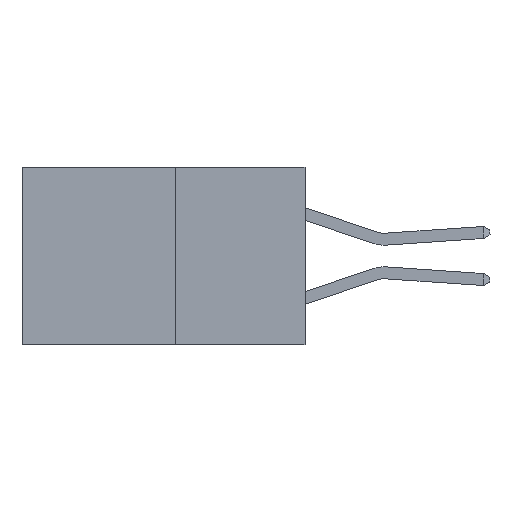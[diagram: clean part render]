
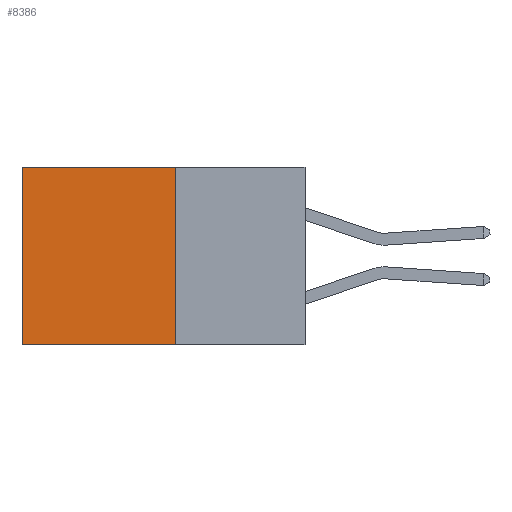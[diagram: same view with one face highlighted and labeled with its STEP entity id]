
A CAD part, left-side view. The second image highlights one B-rep face of the part: STEP entity #8386.
In plain terms, the highlighted planar face has unit normal (-1, 0, 0).
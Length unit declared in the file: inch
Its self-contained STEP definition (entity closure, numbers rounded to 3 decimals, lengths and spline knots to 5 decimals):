
#73 = CARTESIAN_POINT ( 'NONE',  ( 0.277, 0.27, -0.37 ) ) ;
#187 = DIRECTION ( 'NONE',  ( 0., 0., -1. ) ) ;
#1354 = EDGE_CURVE ( 'NONE', #4958, #6235, #5402, .T. ) ;
#1986 = EDGE_CURVE ( 'NONE', #6235, #6941, #6655, .T. ) ;
#2369 = CARTESIAN_POINT ( 'NONE',  ( 0.277, 0.27, -0.37 ) ) ;
#2407 = VECTOR ( 'NONE', #4688, 39.37008 ) ;
#2546 = EDGE_LOOP ( 'NONE', ( #6304, #5049, #4084, #9628 ) ) ;
#2967 = CARTESIAN_POINT ( 'NONE',  ( 0.277, 0.27, 0. ) ) ;
#3850 = CARTESIAN_POINT ( 'NONE',  ( 0.277, 0.27, -0.37 ) ) ;
#3928 = EDGE_CURVE ( 'NONE', #4958, #4453, #10139, .T. ) ;
#3940 = AXIS2_PLACEMENT_3D ( 'NONE', #2369, #4893, #10057 ) ;
#4017 = CARTESIAN_POINT ( 'NONE',  ( 0.277, 0.59, -0.37 ) ) ;
#4084 = ORIENTED_EDGE ( 'NONE', *, *, #1354, .F. ) ;
#4098 = DIRECTION ( 'NONE',  ( 0., 0., -1. ) ) ;
#4453 = VERTEX_POINT ( 'NONE', #5354 ) ;
#4454 = VECTOR ( 'NONE', #7795, 39.37008 ) ;
#4688 = DIRECTION ( 'NONE',  ( 0., 1., 0. ) ) ;
#4707 = EDGE_CURVE ( 'NONE', #4453, #6941, #5083, .T. ) ;
#4893 = DIRECTION ( 'NONE',  ( 1., 0., 0. ) ) ;
#4958 = VERTEX_POINT ( 'NONE', #2967 ) ;
#5049 = ORIENTED_EDGE ( 'NONE', *, *, #1986, .F. ) ;
#5083 = LINE ( 'NONE', #4017, #5330 ) ;
#5199 = CARTESIAN_POINT ( 'NONE',  ( 0.277, 0.27, -0.37 ) ) ;
#5330 = VECTOR ( 'NONE', #4098, 39.37008 ) ;
#5354 = CARTESIAN_POINT ( 'NONE',  ( 0.277, 0.59, 0. ) ) ;
#5402 = LINE ( 'NONE', #5199, #9153 ) ;
#6235 = VERTEX_POINT ( 'NONE', #3850 ) ;
#6304 = ORIENTED_EDGE ( 'NONE', *, *, #4707, .T. ) ;
#6655 = LINE ( 'NONE', #73, #2407 ) ;
#6941 = VERTEX_POINT ( 'NONE', #8971 ) ;
#7795 = DIRECTION ( 'NONE',  ( 0., 1., 0. ) ) ;
#7862 = CARTESIAN_POINT ( 'NONE',  ( 0.277, 0.27, 0. ) ) ;
#8372 = FACE_OUTER_BOUND ( 'NONE', #2546, .T. ) ;
#8386 = ADVANCED_FACE ( 'NONE', ( #8372 ), #9390, .F. ) ;
#8971 = CARTESIAN_POINT ( 'NONE',  ( 0.277, 0.59, -0.37 ) ) ;
#9153 = VECTOR ( 'NONE', #187, 39.37008 ) ;
#9390 = PLANE ( 'NONE',  #3940 ) ;
#9628 = ORIENTED_EDGE ( 'NONE', *, *, #3928, .T. ) ;
#10057 = DIRECTION ( 'NONE',  ( 0., 0., -1. ) ) ;
#10139 = LINE ( 'NONE', #7862, #4454 ) ;
